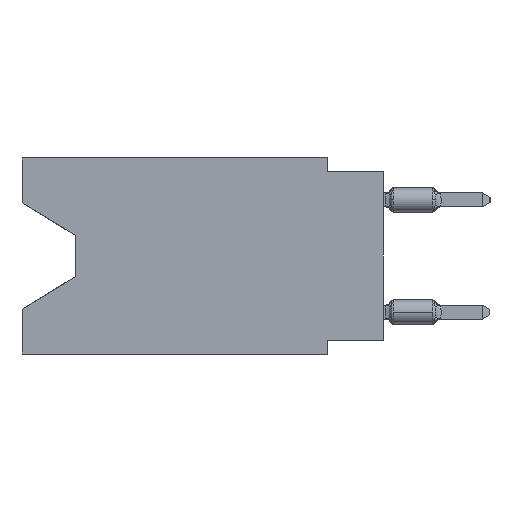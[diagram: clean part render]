
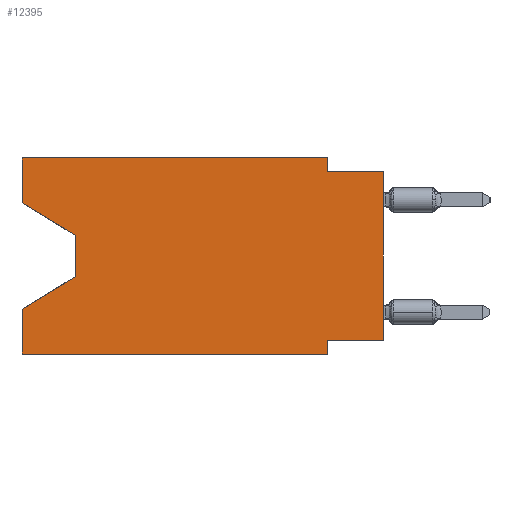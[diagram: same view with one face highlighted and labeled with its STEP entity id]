
A CAD part, left-side view. The second image highlights one B-rep face of the part: STEP entity #12395.
In plain terms, the highlighted planar face has unit normal (-1, 0, 0).
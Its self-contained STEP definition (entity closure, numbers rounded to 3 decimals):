
#593 = DIRECTION ( 'NONE',  ( 1., 0., 0. ) ) ;
#978 = DIRECTION ( 'NONE',  ( 0., 0., -1. ) ) ;
#1132 = ORIENTED_EDGE ( 'NONE', *, *, #12094, .T. ) ;
#1172 = DIRECTION ( 'NONE',  ( 0., -1., 0. ) ) ;
#1433 = VECTOR ( 'NONE', #20450, 1000. ) ;
#1466 = CARTESIAN_POINT ( 'NONE',  ( 0., 16.383, -2.038 ) ) ;
#2390 = VECTOR ( 'NONE', #28230, 1000. ) ;
#2601 = CARTESIAN_POINT ( 'NONE',  ( 0., 0., -0.635 ) ) ;
#3048 = VERTEX_POINT ( 'NONE', #15865 ) ;
#3525 = EDGE_CURVE ( 'NONE', #14915, #4514, #29986, .T. ) ;
#3543 = EDGE_CURVE ( 'NONE', #7111, #3048, #25134, .T. ) ;
#4287 = LINE ( 'NONE', #9656, #1433 ) ;
#4413 = ORIENTED_EDGE ( 'NONE', *, *, #3525, .F. ) ;
#4514 = VERTEX_POINT ( 'NONE', #34441 ) ;
#4621 = EDGE_CURVE ( 'NONE', #6859, #20082, #4287, .T. ) ;
#4746 = DIRECTION ( 'NONE',  ( 0., 0., 1. ) ) ;
#4979 = CARTESIAN_POINT ( 'NONE',  ( 0., 13.97, -5.385 ) ) ;
#5348 = VECTOR ( 'NONE', #10114, 1000. ) ;
#5390 = EDGE_CURVE ( 'NONE', #3048, #28021, #12267, .T. ) ;
#5970 = VECTOR ( 'NONE', #27471, 1000. ) ;
#6665 = VECTOR ( 'NONE', #978, 1000. ) ;
#6859 = VERTEX_POINT ( 'NONE', #23574 ) ;
#6868 = DIRECTION ( 'NONE',  ( 0., 0., -1. ) ) ;
#7111 = VERTEX_POINT ( 'NONE', #1466 ) ;
#7343 = VERTEX_POINT ( 'NONE', #10589 ) ;
#7418 = CARTESIAN_POINT ( 'NONE',  ( 0., 0., -0.635 ) ) ;
#8261 = CARTESIAN_POINT ( 'NONE',  ( 0., 16.383, 0. ) ) ;
#8839 = PLANE ( 'NONE',  #28283 ) ;
#9656 = CARTESIAN_POINT ( 'NONE',  ( 0., 2.54, -8.89 ) ) ;
#10114 = DIRECTION ( 'NONE',  ( 0., 0., 1. ) ) ;
#10332 = VERTEX_POINT ( 'NONE', #32133 ) ;
#10589 = CARTESIAN_POINT ( 'NONE',  ( 0., 2.54, -0.635 ) ) ;
#10935 = LINE ( 'NONE', #16695, #15677 ) ;
#11074 = ORIENTED_EDGE ( 'NONE', *, *, #3543, .T. ) ;
#11349 = CARTESIAN_POINT ( 'NONE',  ( 0., 16.383, 0. ) ) ;
#12066 = EDGE_CURVE ( 'NONE', #7343, #28521, #34729, .T. ) ;
#12094 = EDGE_CURVE ( 'NONE', #16327, #28521, #12468, .T. ) ;
#12107 = CARTESIAN_POINT ( 'NONE',  ( 0., 16.383, -8.89 ) ) ;
#12267 = LINE ( 'NONE', #22693, #6665 ) ;
#12395 = ADVANCED_FACE ( 'NONE', ( #22841 ), #8839, .F. ) ;
#12468 = LINE ( 'NONE', #23417, #5348 ) ;
#13069 = EDGE_CURVE ( 'NONE', #14915, #20082, #17514, .T. ) ;
#13273 = EDGE_CURVE ( 'NONE', #7111, #10332, #20731, .T. ) ;
#13362 = VECTOR ( 'NONE', #14986, 1000. ) ;
#13605 = EDGE_CURVE ( 'NONE', #10332, #18775, #30933, .T. ) ;
#14027 = LINE ( 'NONE', #14375, #26591 ) ;
#14375 = CARTESIAN_POINT ( 'NONE',  ( 0., 0., -8.255 ) ) ;
#14673 = ORIENTED_EDGE ( 'NONE', *, *, #20429, .T. ) ;
#14793 = EDGE_CURVE ( 'NONE', #18775, #7343, #18012, .T. ) ;
#14915 = VERTEX_POINT ( 'NONE', #32175 ) ;
#14986 = DIRECTION ( 'NONE',  ( 0., -1., 0. ) ) ;
#15677 = VECTOR ( 'NONE', #30704, 1000. ) ;
#15865 = CARTESIAN_POINT ( 'NONE',  ( 0., 13.97, -3.505 ) ) ;
#16088 = ORIENTED_EDGE ( 'NONE', *, *, #14793, .F. ) ;
#16327 = VERTEX_POINT ( 'NONE', #18346 ) ;
#16695 = CARTESIAN_POINT ( 'NONE',  ( 0., 13.97, -5.385 ) ) ;
#17174 = ORIENTED_EDGE ( 'NONE', *, *, #12066, .F. ) ;
#17285 = CARTESIAN_POINT ( 'NONE',  ( 0., 16.383, 0. ) ) ;
#17514 = LINE ( 'NONE', #12107, #21864 ) ;
#17866 = CARTESIAN_POINT ( 'NONE',  ( 0., 2.54, 0. ) ) ;
#18012 = LINE ( 'NONE', #28591, #18187 ) ;
#18187 = VECTOR ( 'NONE', #6868, 1000. ) ;
#18346 = CARTESIAN_POINT ( 'NONE',  ( 0., 0., -8.255 ) ) ;
#18770 = ORIENTED_EDGE ( 'NONE', *, *, #4621, .F. ) ;
#18775 = VERTEX_POINT ( 'NONE', #17866 ) ;
#20082 = VERTEX_POINT ( 'NONE', #23368 ) ;
#20429 = EDGE_CURVE ( 'NONE', #28021, #4514, #10935, .T. ) ;
#20450 = DIRECTION ( 'NONE',  ( 0., 0., -1. ) ) ;
#20731 = LINE ( 'NONE', #25933, #25889 ) ;
#21679 = ORIENTED_EDGE ( 'NONE', *, *, #13273, .F. ) ;
#21864 = VECTOR ( 'NONE', #1172, 1000. ) ;
#22139 = DIRECTION ( 'NONE',  ( 0., 0., -1. ) ) ;
#22693 = CARTESIAN_POINT ( 'NONE',  ( 0., 13.97, -3.505 ) ) ;
#22841 = FACE_OUTER_BOUND ( 'NONE', #31456, .T. ) ;
#23368 = CARTESIAN_POINT ( 'NONE',  ( 0., 2.54, -8.89 ) ) ;
#23417 = CARTESIAN_POINT ( 'NONE',  ( 0., 0., 0. ) ) ;
#23574 = CARTESIAN_POINT ( 'NONE',  ( 0., 2.54, -8.255 ) ) ;
#24436 = ORIENTED_EDGE ( 'NONE', *, *, #13605, .F. ) ;
#24768 = CARTESIAN_POINT ( 'NONE',  ( 0., 16.383, -2.038 ) ) ;
#25134 = LINE ( 'NONE', #24768, #5970 ) ;
#25315 = DIRECTION ( 'NONE',  ( 0., 1., 0. ) ) ;
#25559 = ORIENTED_EDGE ( 'NONE', *, *, #5390, .T. ) ;
#25889 = VECTOR ( 'NONE', #4746, 1000. ) ;
#25933 = CARTESIAN_POINT ( 'NONE',  ( 0., 16.383, 0. ) ) ;
#26591 = VECTOR ( 'NONE', #25315, 1000. ) ;
#26606 = VECTOR ( 'NONE', #30518, 1000. ) ;
#27471 = DIRECTION ( 'NONE',  ( 0., -0.855, -0.519 ) ) ;
#28021 = VERTEX_POINT ( 'NONE', #4979 ) ;
#28230 = DIRECTION ( 'NONE',  ( 0., -1., 0. ) ) ;
#28283 = AXIS2_PLACEMENT_3D ( 'NONE', #11349, #593, #22139 ) ;
#28521 = VERTEX_POINT ( 'NONE', #2601 ) ;
#28591 = CARTESIAN_POINT ( 'NONE',  ( 0., 2.54, 0. ) ) ;
#29986 = LINE ( 'NONE', #8261, #26606 ) ;
#30518 = DIRECTION ( 'NONE',  ( 0., 0., 1. ) ) ;
#30704 = DIRECTION ( 'NONE',  ( 0., 0.855, -0.519 ) ) ;
#30933 = LINE ( 'NONE', #17285, #2390 ) ;
#31456 = EDGE_LOOP ( 'NONE', ( #11074, #25559, #14673, #4413, #32051, #18770, #34766, #1132, #17174, #16088, #24436, #21679 ) ) ;
#32051 = ORIENTED_EDGE ( 'NONE', *, *, #13069, .T. ) ;
#32133 = CARTESIAN_POINT ( 'NONE',  ( 0., 16.383, 0. ) ) ;
#32175 = CARTESIAN_POINT ( 'NONE',  ( 0., 16.383, -8.89 ) ) ;
#33881 = EDGE_CURVE ( 'NONE', #16327, #6859, #14027, .T. ) ;
#34441 = CARTESIAN_POINT ( 'NONE',  ( 0., 16.383, -6.852 ) ) ;
#34729 = LINE ( 'NONE', #7418, #13362 ) ;
#34766 = ORIENTED_EDGE ( 'NONE', *, *, #33881, .F. ) ;
